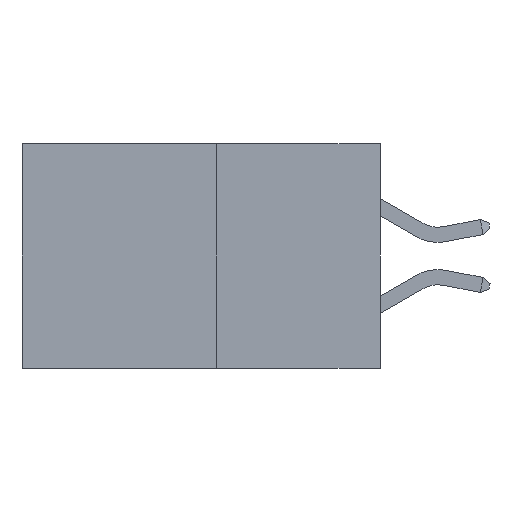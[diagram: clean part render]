
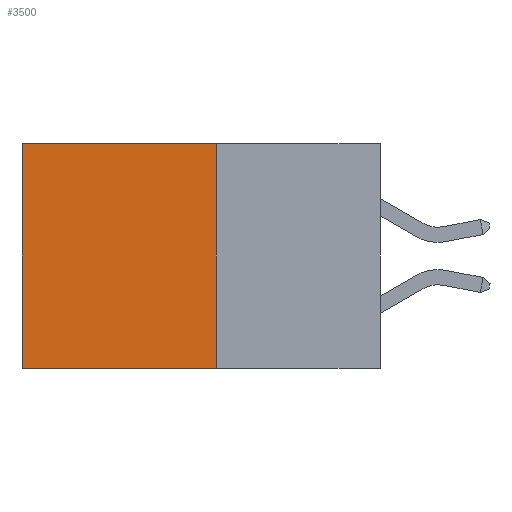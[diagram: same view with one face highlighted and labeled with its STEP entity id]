
A CAD part, left-side view. The second image highlights one B-rep face of the part: STEP entity #3500.
In plain terms, the highlighted planar face has unit normal (-1, 0, 0).
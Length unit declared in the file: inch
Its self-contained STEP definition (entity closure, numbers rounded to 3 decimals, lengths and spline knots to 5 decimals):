
#353 = ORIENTED_EDGE ( 'NONE', *, *, #10416, .T. ) ;
#400 = LINE ( 'NONE', #8787, #4585 ) ;
#634 = CARTESIAN_POINT ( 'NONE',  ( 0.277, 0.27, -0.37 ) ) ;
#659 = EDGE_LOOP ( 'NONE', ( #2614, #7499, #816, #353 ) ) ;
#816 = ORIENTED_EDGE ( 'NONE', *, *, #7447, .F. ) ;
#1187 = DIRECTION ( 'NONE',  ( 0., 1., 0. ) ) ;
#1304 = VECTOR ( 'NONE', #7814, 39.37008 ) ;
#1438 = CARTESIAN_POINT ( 'NONE',  ( 0.277, 0.27, -0.37 ) ) ;
#1491 = VERTEX_POINT ( 'NONE', #4204 ) ;
#2362 = AXIS2_PLACEMENT_3D ( 'NONE', #1438, #4762, #10497 ) ;
#2614 = ORIENTED_EDGE ( 'NONE', *, *, #4646, .T. ) ;
#2761 = EDGE_CURVE ( 'NONE', #8927, #4042, #3800, .T. ) ;
#3461 = DIRECTION ( 'NONE',  ( 0., 0., -1. ) ) ;
#3500 = ADVANCED_FACE ( 'NONE', ( #7796 ), #7228, .F. ) ;
#3783 = CARTESIAN_POINT ( 'NONE',  ( 0.277, 0.59, -0.37 ) ) ;
#3800 = LINE ( 'NONE', #634, #10350 ) ;
#4042 = VERTEX_POINT ( 'NONE', #3783 ) ;
#4204 = CARTESIAN_POINT ( 'NONE',  ( 0.277, 0.27, 0. ) ) ;
#4494 = CARTESIAN_POINT ( 'NONE',  ( 0.277, 0.27, 0. ) ) ;
#4585 = VECTOR ( 'NONE', #8017, 39.37008 ) ;
#4646 = EDGE_CURVE ( 'NONE', #9567, #4042, #5163, .T. ) ;
#4762 = DIRECTION ( 'NONE',  ( 1., 0., 0. ) ) ;
#4908 = VECTOR ( 'NONE', #3461, 39.37008 ) ;
#5163 = LINE ( 'NONE', #6712, #4908 ) ;
#6712 = CARTESIAN_POINT ( 'NONE',  ( 0.277, 0.59, -0.37 ) ) ;
#6990 = CARTESIAN_POINT ( 'NONE',  ( 0.277, 0.27, -0.37 ) ) ;
#7228 = PLANE ( 'NONE',  #2362 ) ;
#7447 = EDGE_CURVE ( 'NONE', #1491, #8927, #400, .T. ) ;
#7499 = ORIENTED_EDGE ( 'NONE', *, *, #2761, .F. ) ;
#7793 = CARTESIAN_POINT ( 'NONE',  ( 0.277, 0.59, 0. ) ) ;
#7796 = FACE_OUTER_BOUND ( 'NONE', #659, .T. ) ;
#7814 = DIRECTION ( 'NONE',  ( 0., 1., 0. ) ) ;
#8017 = DIRECTION ( 'NONE',  ( 0., 0., -1. ) ) ;
#8787 = CARTESIAN_POINT ( 'NONE',  ( 0.277, 0.27, -0.37 ) ) ;
#8927 = VERTEX_POINT ( 'NONE', #6990 ) ;
#9567 = VERTEX_POINT ( 'NONE', #7793 ) ;
#10328 = LINE ( 'NONE', #4494, #1304 ) ;
#10350 = VECTOR ( 'NONE', #1187, 39.37008 ) ;
#10416 = EDGE_CURVE ( 'NONE', #1491, #9567, #10328, .T. ) ;
#10497 = DIRECTION ( 'NONE',  ( 0., 0., -1. ) ) ;
